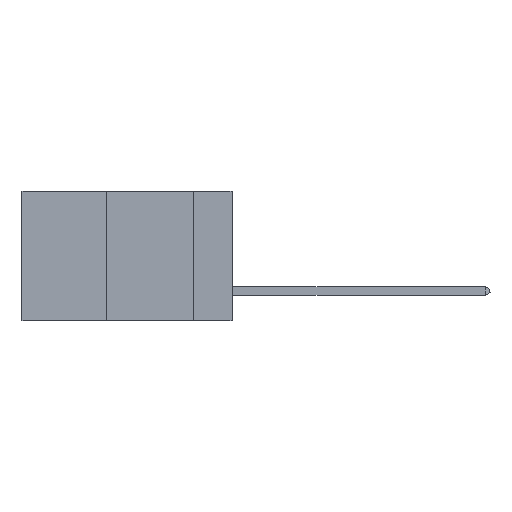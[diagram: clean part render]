
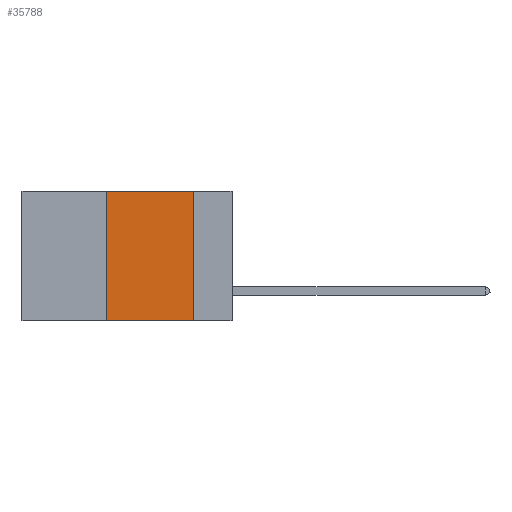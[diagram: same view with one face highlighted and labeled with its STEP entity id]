
A CAD part, left-side view. The second image highlights one B-rep face of the part: STEP entity #35788.
In plain terms, the highlighted planar face has unit normal (-1, 0, 0).
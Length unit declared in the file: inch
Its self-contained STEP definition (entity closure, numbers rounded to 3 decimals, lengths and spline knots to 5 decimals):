
#115 = FACE_OUTER_BOUND ( 'NONE', #868, .T. ) ;
#868 = EDGE_LOOP ( 'NONE', ( #13603, #7197, #2262, #36303 ) ) ;
#2262 = ORIENTED_EDGE ( 'NONE', *, *, #3068, .F. ) ;
#3068 = EDGE_CURVE ( 'NONE', #33450, #29486, #20039, .T. ) ;
#3424 = LINE ( 'NONE', #16754, #22800 ) ;
#7197 = ORIENTED_EDGE ( 'NONE', *, *, #17084, .F. ) ;
#7198 = CARTESIAN_POINT ( 'NONE',  ( 0., 0.6, 0. ) ) ;
#7497 = AXIS2_PLACEMENT_3D ( 'NONE', #7198, #9586, #29954 ) ;
#8141 = CARTESIAN_POINT ( 'NONE',  ( 0., 0.36, -0.37 ) ) ;
#9586 = DIRECTION ( 'NONE',  ( 1., 0., 0. ) ) ;
#10113 = DIRECTION ( 'NONE',  ( 0., 0., 1. ) ) ;
#10129 = LINE ( 'NONE', #10780, #28581 ) ;
#10168 = EDGE_CURVE ( 'NONE', #34403, #24358, #21631, .T. ) ;
#10780 = CARTESIAN_POINT ( 'NONE',  ( 0., 0.6, -0.37 ) ) ;
#11489 = CARTESIAN_POINT ( 'NONE',  ( 0., 0.11, 0. ) ) ;
#12849 = PLANE ( 'NONE',  #7497 ) ;
#13396 = CARTESIAN_POINT ( 'NONE',  ( 0., 0.36, 0. ) ) ;
#13603 = ORIENTED_EDGE ( 'NONE', *, *, #10168, .F. ) ;
#14228 = DIRECTION ( 'NONE',  ( 0., 0., -1. ) ) ;
#14471 = CARTESIAN_POINT ( 'NONE',  ( 0., 0.11, 0. ) ) ;
#16754 = CARTESIAN_POINT ( 'NONE',  ( 0., 0.6, 0. ) ) ;
#17084 = EDGE_CURVE ( 'NONE', #29486, #34403, #3424, .T. ) ;
#19010 = CARTESIAN_POINT ( 'NONE',  ( 0., 0.36, 0. ) ) ;
#20039 = LINE ( 'NONE', #19010, #27704 ) ;
#21631 = LINE ( 'NONE', #14471, #22536 ) ;
#21930 = DIRECTION ( 'NONE',  ( 0., -1., 0. ) ) ;
#22475 = CARTESIAN_POINT ( 'NONE',  ( 0., 0.11, -0.37 ) ) ;
#22536 = VECTOR ( 'NONE', #14228, 39.37008 ) ;
#22800 = VECTOR ( 'NONE', #31351, 39.37008 ) ;
#24358 = VERTEX_POINT ( 'NONE', #22475 ) ;
#27704 = VECTOR ( 'NONE', #10113, 39.37008 ) ;
#28581 = VECTOR ( 'NONE', #21930, 39.37008 ) ;
#29409 = EDGE_CURVE ( 'NONE', #33450, #24358, #10129, .T. ) ;
#29486 = VERTEX_POINT ( 'NONE', #13396 ) ;
#29954 = DIRECTION ( 'NONE',  ( 0., 0., -1. ) ) ;
#31351 = DIRECTION ( 'NONE',  ( 0., -1., 0. ) ) ;
#33450 = VERTEX_POINT ( 'NONE', #8141 ) ;
#34403 = VERTEX_POINT ( 'NONE', #11489 ) ;
#35788 = ADVANCED_FACE ( 'NONE', ( #115 ), #12849, .F. ) ;
#36303 = ORIENTED_EDGE ( 'NONE', *, *, #29409, .T. ) ;
